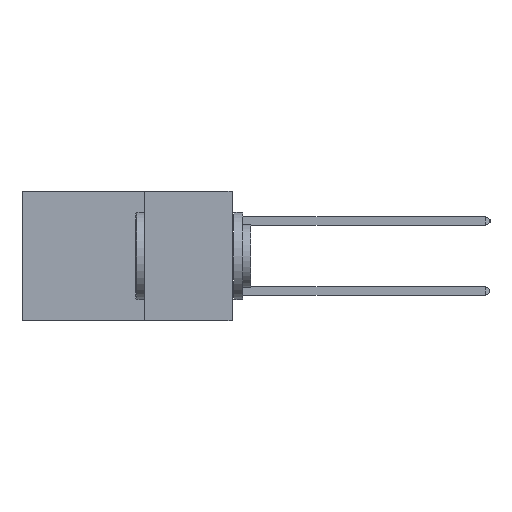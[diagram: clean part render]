
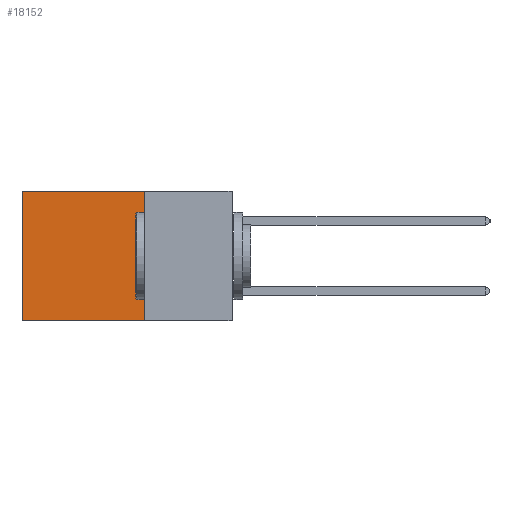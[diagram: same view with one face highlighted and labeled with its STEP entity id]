
A CAD part, left-side view. The second image highlights one B-rep face of the part: STEP entity #18152.
In plain terms, the highlighted planar face has unit normal (-1, 0, 0).
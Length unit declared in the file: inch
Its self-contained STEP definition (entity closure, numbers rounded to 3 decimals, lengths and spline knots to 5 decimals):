
#508 = DIRECTION ( 'NONE',  ( 0., 0., -1. ) ) ;
#1918 = CARTESIAN_POINT ( 'NONE',  ( 0.2875, 0.25, -0.37 ) ) ;
#2269 = LINE ( 'NONE', #21609, #20637 ) ;
#2339 = ORIENTED_EDGE ( 'NONE', *, *, #6338, .T. ) ;
#4130 = DIRECTION ( 'NONE',  ( 0., 1., 0. ) ) ;
#4224 = EDGE_CURVE ( 'NONE', #22523, #6937, #2269, .T. ) ;
#4525 = ORIENTED_EDGE ( 'NONE', *, *, #4224, .T. ) ;
#5145 = PLANE ( 'NONE',  #12044 ) ;
#5274 = CARTESIAN_POINT ( 'NONE',  ( 0.2875, 0.6, 0. ) ) ;
#5506 = DIRECTION ( 'NONE',  ( 0., 1., 0. ) ) ;
#5572 = CARTESIAN_POINT ( 'NONE',  ( 0.2875, 0.6, 0. ) ) ;
#5804 = EDGE_CURVE ( 'NONE', #13979, #9200, #20032, .T. ) ;
#6338 = EDGE_CURVE ( 'NONE', #6937, #9200, #20260, .T. ) ;
#6406 = VECTOR ( 'NONE', #9160, 39.37008 ) ;
#6937 = VERTEX_POINT ( 'NONE', #5274 ) ;
#7008 = DIRECTION ( 'NONE',  ( 0., 0., -1. ) ) ;
#8314 = CARTESIAN_POINT ( 'NONE',  ( 0.2875, 0.6, -0.37 ) ) ;
#8817 = FACE_OUTER_BOUND ( 'NONE', #19881, .T. ) ;
#9160 = DIRECTION ( 'NONE',  ( 0., 0., -1. ) ) ;
#9200 = VERTEX_POINT ( 'NONE', #8314 ) ;
#10854 = VECTOR ( 'NONE', #508, 39.37008 ) ;
#11929 = ORIENTED_EDGE ( 'NONE', *, *, #22288, .F. ) ;
#12044 = AXIS2_PLACEMENT_3D ( 'NONE', #22481, #17469, #7008 ) ;
#13269 = CARTESIAN_POINT ( 'NONE',  ( 0.2875, 0.25, 0. ) ) ;
#13979 = VERTEX_POINT ( 'NONE', #1918 ) ;
#15465 = VECTOR ( 'NONE', #5506, 39.37008 ) ;
#15501 = LINE ( 'NONE', #13269, #10854 ) ;
#15700 = ORIENTED_EDGE ( 'NONE', *, *, #5804, .F. ) ;
#17469 = DIRECTION ( 'NONE',  ( 1., 0., 0. ) ) ;
#17791 = CARTESIAN_POINT ( 'NONE',  ( 0.2875, 0.25, -0.37 ) ) ;
#18152 = ADVANCED_FACE ( 'NONE', ( #8817 ), #5145, .F. ) ;
#18318 = CARTESIAN_POINT ( 'NONE',  ( 0.2875, 0.25, 0. ) ) ;
#19881 = EDGE_LOOP ( 'NONE', ( #2339, #15700, #11929, #4525 ) ) ;
#20032 = LINE ( 'NONE', #17791, #15465 ) ;
#20260 = LINE ( 'NONE', #5572, #6406 ) ;
#20637 = VECTOR ( 'NONE', #4130, 39.37008 ) ;
#21609 = CARTESIAN_POINT ( 'NONE',  ( 0.2875, 0.25, 0. ) ) ;
#22288 = EDGE_CURVE ( 'NONE', #22523, #13979, #15501, .T. ) ;
#22481 = CARTESIAN_POINT ( 'NONE',  ( 0.2875, 0.25, 0. ) ) ;
#22523 = VERTEX_POINT ( 'NONE', #18318 ) ;
